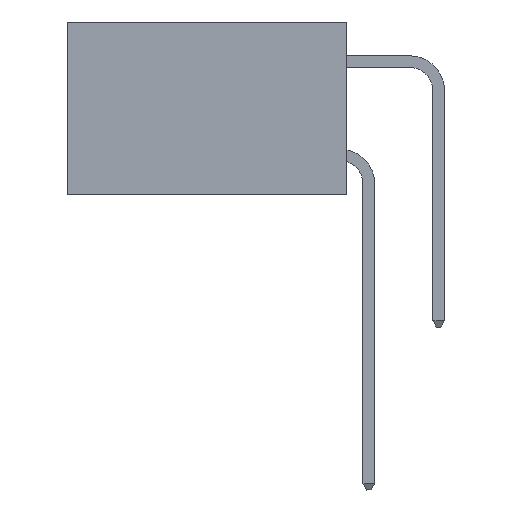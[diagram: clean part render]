
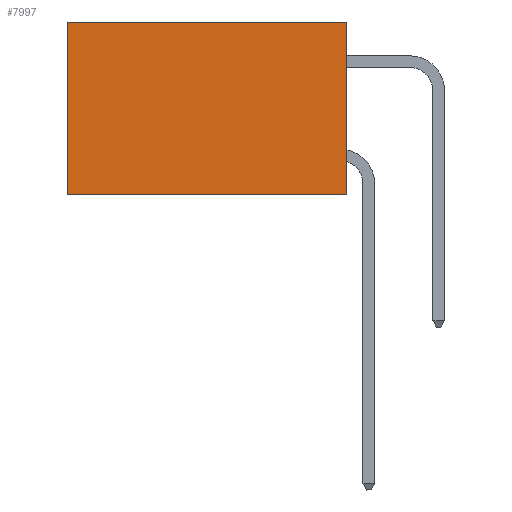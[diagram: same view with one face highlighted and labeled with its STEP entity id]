
A CAD part, left-side view. The second image highlights one B-rep face of the part: STEP entity #7997.
In plain terms, the highlighted planar face has unit normal (-1, 0, 0).
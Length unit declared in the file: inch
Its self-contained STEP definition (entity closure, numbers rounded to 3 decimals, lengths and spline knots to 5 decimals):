
#207 = DIRECTION ( 'NONE',  ( 0., 0., -1. ) ) ;
#461 = VECTOR ( 'NONE', #3756, 39.37008 ) ;
#1244 = PLANE ( 'NONE',  #11350 ) ;
#1321 = FACE_OUTER_BOUND ( 'NONE', #1632, .T. ) ;
#1489 = LINE ( 'NONE', #9101, #8238 ) ;
#1588 = VERTEX_POINT ( 'NONE', #2394 ) ;
#1632 = EDGE_LOOP ( 'NONE', ( #2127, #2149, #2177, #2199 ) ) ;
#2022 = DIRECTION ( 'NONE',  ( 0., 1., 0. ) ) ;
#2127 = ORIENTED_EDGE ( 'NONE', *, *, #9057, .T. ) ;
#2149 = ORIENTED_EDGE ( 'NONE', *, *, #3444, .F. ) ;
#2177 = ORIENTED_EDGE ( 'NONE', *, *, #7862, .F. ) ;
#2199 = ORIENTED_EDGE ( 'NONE', *, *, #4631, .T. ) ;
#2394 = CARTESIAN_POINT ( 'NONE',  ( 0.2875, 0.6, 0. ) ) ;
#2753 = VECTOR ( 'NONE', #2022, 39.37008 ) ;
#3016 = LINE ( 'NONE', #4379, #5290 ) ;
#3208 = VERTEX_POINT ( 'NONE', #5382 ) ;
#3379 = LINE ( 'NONE', #7868, #2753 ) ;
#3444 = EDGE_CURVE ( 'NONE', #7313, #3208, #3379, .T. ) ;
#3756 = DIRECTION ( 'NONE',  ( 0., 1., 0. ) ) ;
#3955 = CARTESIAN_POINT ( 'NONE',  ( 0.2875, 0., 0. ) ) ;
#4379 = CARTESIAN_POINT ( 'NONE',  ( 0.2875, 0.6, 0. ) ) ;
#4631 = EDGE_CURVE ( 'NONE', #10532, #1588, #10325, .T. ) ;
#5217 = CARTESIAN_POINT ( 'NONE',  ( 0.2875, 0., 0. ) ) ;
#5290 = VECTOR ( 'NONE', #9413, 39.37008 ) ;
#5382 = CARTESIAN_POINT ( 'NONE',  ( 0.2875, 0.6, -0.37 ) ) ;
#6095 = DIRECTION ( 'NONE',  ( 1., 0., 0. ) ) ;
#6266 = CARTESIAN_POINT ( 'NONE',  ( 0.2875, 0., 0. ) ) ;
#7313 = VERTEX_POINT ( 'NONE', #8298 ) ;
#7862 = EDGE_CURVE ( 'NONE', #10532, #7313, #1489, .T. ) ;
#7868 = CARTESIAN_POINT ( 'NONE',  ( 0.2875, 0., -0.37 ) ) ;
#7997 = ADVANCED_FACE ( 'NONE', ( #1321 ), #1244, .F. ) ;
#8238 = VECTOR ( 'NONE', #11521, 39.37008 ) ;
#8298 = CARTESIAN_POINT ( 'NONE',  ( 0.2875, 0., -0.37 ) ) ;
#9057 = EDGE_CURVE ( 'NONE', #1588, #3208, #3016, .T. ) ;
#9101 = CARTESIAN_POINT ( 'NONE',  ( 0.2875, 0., 0. ) ) ;
#9413 = DIRECTION ( 'NONE',  ( 0., 0., -1. ) ) ;
#10325 = LINE ( 'NONE', #3955, #461 ) ;
#10532 = VERTEX_POINT ( 'NONE', #6266 ) ;
#11350 = AXIS2_PLACEMENT_3D ( 'NONE', #5217, #6095, #207 ) ;
#11521 = DIRECTION ( 'NONE',  ( 0., 0., -1. ) ) ;
